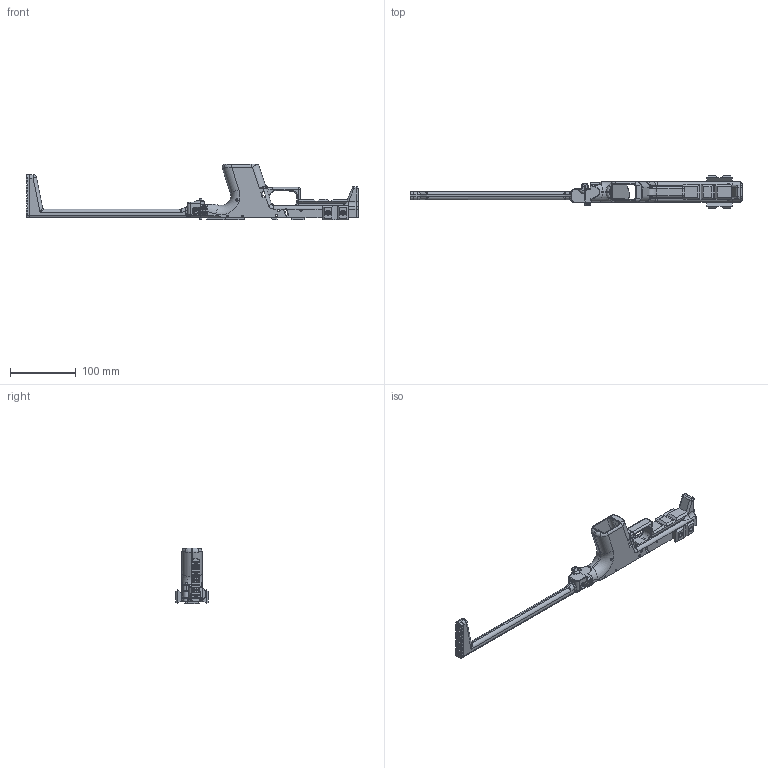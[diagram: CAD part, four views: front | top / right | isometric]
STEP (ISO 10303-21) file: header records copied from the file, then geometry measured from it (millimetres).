
FILE_DESCRIPTION(/* description */ (''),/* implementation_level */ '2;1');
FILE_NAME(/* name */ 'p80 PDW V2.stp',/* time_stamp */ '2019-12-27T01:16:59+02:00',/* author */ (''),/* organization */ (''),/* preprocessor_version */ 'ST-DEVELOPER v15.2',/* originating_system */ 'Autodesk Translator Framework v2.0.0.5431',/* authorisation */ '');
FILE_SCHEMA (('AUTOMOTIVE_DESIGN { 1 0 10303 214 3 1 1 }'));
Length unit declared in the file: centimetre
Products named in the file (1): GLOCK PDW V4 WITH RAILS
Bounding box: 506.63 x 49.6 x 85.41 mm (x, y, z)
Volume: 214816.8 mm3; surface area: 113189.4 mm2
Topology: 17 solids, 17 shells, 1673 faces, 4287 edges, 2597 vertices
Faces by surface type: plane 673, cylinder 493, bspline 267, torus 125, cone 69, sphere 46
Full cylindrical faces by diameter (mm): 1.25 x8, 1.655 x8, 1.8 x1, 2.5 x9, 3.057 x4, 3.06 x3, 3.675 x4, 4 x3, 4.042 x2, 6.5 x1, 6.825 x4, 7.2 x1, 7.4 x1, 8 x1, 9 x1
Entity records: 56823 total; most frequent: CARTESIAN_POINT 17751, ORIENTED_EDGE 8260, DIRECTION 7868, EDGE_CURVE 4130, AXIS2_PLACEMENT_3D 2847, VERTEX_POINT 2573, LINE 2174, VECTOR 2174
